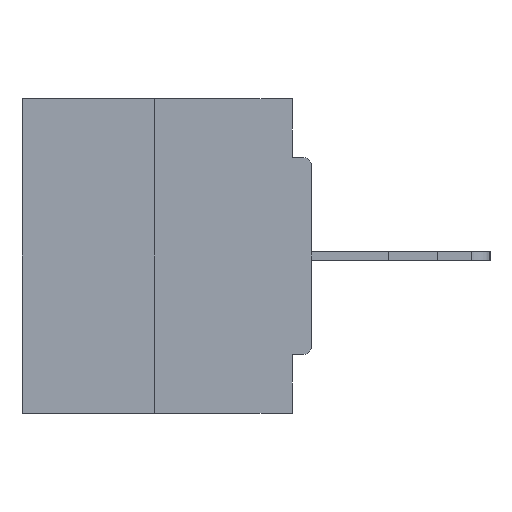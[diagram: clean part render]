
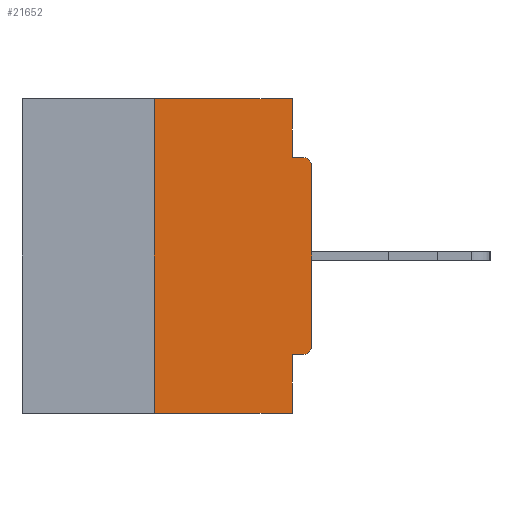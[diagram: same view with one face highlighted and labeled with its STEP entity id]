
A CAD part, left-side view. The second image highlights one B-rep face of the part: STEP entity #21652.
In plain terms, the highlighted planar face has unit normal (-1, 0, 0).
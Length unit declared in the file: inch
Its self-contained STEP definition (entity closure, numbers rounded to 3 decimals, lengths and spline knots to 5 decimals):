
#1055 = DIRECTION ( 'NONE',  ( 0., 0., -1. ) ) ;
#1206 = CARTESIAN_POINT ( 'NONE',  ( 0., 0.031, 0. ) ) ;
#1295 = DIRECTION ( 'NONE',  ( -1., 0., 0. ) ) ;
#1428 = ORIENTED_EDGE ( 'NONE', *, *, #10351, .T. ) ;
#1651 = VERTEX_POINT ( 'NONE', #8715 ) ;
#1742 = VERTEX_POINT ( 'NONE', #6237 ) ;
#2087 = AXIS2_PLACEMENT_3D ( 'NONE', #4057, #1295, #6509 ) ;
#2750 = LINE ( 'NONE', #12156, #12181 ) ;
#2859 = EDGE_CURVE ( 'NONE', #8785, #9947, #6772, .T. ) ;
#2908 = DIRECTION ( 'NONE',  ( 1., 0., 0. ) ) ;
#3377 = LINE ( 'NONE', #1206, #12599 ) ;
#3978 = CARTESIAN_POINT ( 'NONE',  ( 0., 0.46, 0. ) ) ;
#4057 = CARTESIAN_POINT ( 'NONE',  ( 0., 0.015, -0.3915 ) ) ;
#4497 = DIRECTION ( 'NONE',  ( -1., 0., 0. ) ) ;
#5655 = CARTESIAN_POINT ( 'NONE',  ( 0., 0., -0.3915 ) ) ;
#6237 = CARTESIAN_POINT ( 'NONE',  ( 0., 0.25, 0. ) ) ;
#6465 = ORIENTED_EDGE ( 'NONE', *, *, #26402, .F. ) ;
#6509 = DIRECTION ( 'NONE',  ( 0., 0., -1. ) ) ;
#6772 = LINE ( 'NONE', #21590, #23775 ) ;
#7072 = EDGE_CURVE ( 'NONE', #29787, #1742, #25748, .T. ) ;
#7331 = ORIENTED_EDGE ( 'NONE', *, *, #30289, .T. ) ;
#7629 = VECTOR ( 'NONE', #18260, 39.37008 ) ;
#8656 = ORIENTED_EDGE ( 'NONE', *, *, #25622, .F. ) ;
#8664 = ORIENTED_EDGE ( 'NONE', *, *, #28635, .F. ) ;
#8678 = CIRCLE ( 'NONE', #11634, 0.015 ) ;
#8715 = CARTESIAN_POINT ( 'NONE',  ( 0., 0.015, -0.4065 ) ) ;
#8785 = VERTEX_POINT ( 'NONE', #5655 ) ;
#9453 = CARTESIAN_POINT ( 'NONE',  ( 0., 0.25, -0.5 ) ) ;
#9947 = VERTEX_POINT ( 'NONE', #20185 ) ;
#10351 = EDGE_CURVE ( 'NONE', #1651, #8785, #28680, .T. ) ;
#10397 = ORIENTED_EDGE ( 'NONE', *, *, #28811, .F. ) ;
#11634 = AXIS2_PLACEMENT_3D ( 'NONE', #13630, #4497, #21020 ) ;
#12027 = CARTESIAN_POINT ( 'NONE',  ( 0., 0.25, 0. ) ) ;
#12115 = ORIENTED_EDGE ( 'NONE', *, *, #7072, .F. ) ;
#12156 = CARTESIAN_POINT ( 'NONE',  ( 0., 0.46, -0.5 ) ) ;
#12181 = VECTOR ( 'NONE', #23407, 39.37008 ) ;
#12310 = DIRECTION ( 'NONE',  ( 0., 0., -1. ) ) ;
#12599 = VECTOR ( 'NONE', #1055, 39.37008 ) ;
#13386 = DIRECTION ( 'NONE',  ( 0., -1., 0. ) ) ;
#13630 = CARTESIAN_POINT ( 'NONE',  ( 0., 0.015, -0.1085 ) ) ;
#14059 = CARTESIAN_POINT ( 'NONE',  ( 0., 0.031, -0.5 ) ) ;
#14277 = VERTEX_POINT ( 'NONE', #23774 ) ;
#14624 = CARTESIAN_POINT ( 'NONE',  ( 0., 0.031, -0.0935 ) ) ;
#14626 = VERTEX_POINT ( 'NONE', #18812 ) ;
#15367 = EDGE_LOOP ( 'NONE', ( #10397, #12115, #7331, #16145, #6465, #1428, #22298, #21107, #8656, #8664 ) ) ;
#15702 = LINE ( 'NONE', #3978, #19492 ) ;
#15837 = CARTESIAN_POINT ( 'NONE',  ( 0., 0.031, -0.5 ) ) ;
#16066 = VECTOR ( 'NONE', #16663, 39.37008 ) ;
#16071 = DIRECTION ( 'NONE',  ( 0., -1., 0. ) ) ;
#16145 = ORIENTED_EDGE ( 'NONE', *, *, #21752, .F. ) ;
#16663 = DIRECTION ( 'NONE',  ( 0., 0., 1. ) ) ;
#17892 = VECTOR ( 'NONE', #29428, 39.37008 ) ;
#18260 = DIRECTION ( 'NONE',  ( 0., 1., 0. ) ) ;
#18406 = VERTEX_POINT ( 'NONE', #14624 ) ;
#18444 = CARTESIAN_POINT ( 'NONE',  ( 0., 0.031, 0. ) ) ;
#18580 = LINE ( 'NONE', #21048, #7629 ) ;
#18688 = CARTESIAN_POINT ( 'NONE',  ( 0., 0., -0.0935 ) ) ;
#18812 = CARTESIAN_POINT ( 'NONE',  ( 0., 0.031, -0.4065 ) ) ;
#19257 = PLANE ( 'NONE',  #27270 ) ;
#19492 = VECTOR ( 'NONE', #13386, 39.37008 ) ;
#20164 = LINE ( 'NONE', #15837, #17892 ) ;
#20185 = CARTESIAN_POINT ( 'NONE',  ( 0., 0., -0.1085 ) ) ;
#21020 = DIRECTION ( 'NONE',  ( 0., 0., -1. ) ) ;
#21048 = CARTESIAN_POINT ( 'NONE',  ( 0., 0., -0.4065 ) ) ;
#21107 = ORIENTED_EDGE ( 'NONE', *, *, #23924, .T. ) ;
#21590 = CARTESIAN_POINT ( 'NONE',  ( 0., 0., 0. ) ) ;
#21652 = ADVANCED_FACE ( 'NONE', ( #28804 ), #19257, .F. ) ;
#21752 = EDGE_CURVE ( 'NONE', #14626, #25796, #20164, .T. ) ;
#22298 = ORIENTED_EDGE ( 'NONE', *, *, #2859, .T. ) ;
#23011 = LINE ( 'NONE', #18688, #28896 ) ;
#23407 = DIRECTION ( 'NONE',  ( 0., -1., 0. ) ) ;
#23724 = DIRECTION ( 'NONE',  ( 0., 0., 1. ) ) ;
#23774 = CARTESIAN_POINT ( 'NONE',  ( 0., 0.015, -0.0935 ) ) ;
#23775 = VECTOR ( 'NONE', #23724, 39.37008 ) ;
#23924 = EDGE_CURVE ( 'NONE', #9947, #14277, #8678, .T. ) ;
#24031 = CARTESIAN_POINT ( 'NONE',  ( 0., 0.46, 0. ) ) ;
#25622 = EDGE_CURVE ( 'NONE', #18406, #14277, #23011, .T. ) ;
#25748 = LINE ( 'NONE', #12027, #16066 ) ;
#25796 = VERTEX_POINT ( 'NONE', #14059 ) ;
#26402 = EDGE_CURVE ( 'NONE', #1651, #14626, #18580, .T. ) ;
#27270 = AXIS2_PLACEMENT_3D ( 'NONE', #24031, #2908, #12310 ) ;
#28635 = EDGE_CURVE ( 'NONE', #30431, #18406, #3377, .T. ) ;
#28680 = CIRCLE ( 'NONE', #2087, 0.015 ) ;
#28804 = FACE_OUTER_BOUND ( 'NONE', #15367, .T. ) ;
#28811 = EDGE_CURVE ( 'NONE', #1742, #30431, #15702, .T. ) ;
#28896 = VECTOR ( 'NONE', #16071, 39.37008 ) ;
#29428 = DIRECTION ( 'NONE',  ( 0., 0., -1. ) ) ;
#29787 = VERTEX_POINT ( 'NONE', #9453 ) ;
#30289 = EDGE_CURVE ( 'NONE', #29787, #25796, #2750, .T. ) ;
#30431 = VERTEX_POINT ( 'NONE', #18444 ) ;
